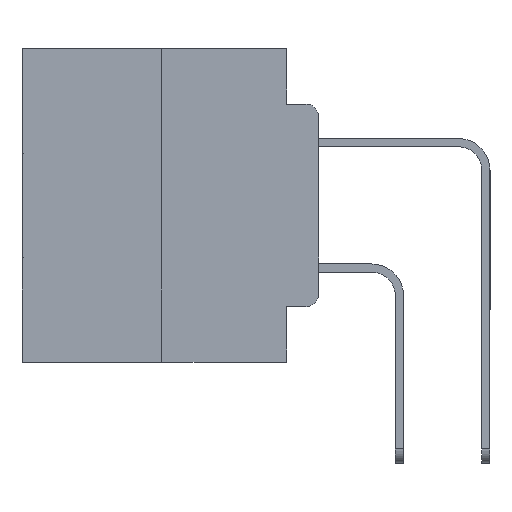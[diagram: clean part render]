
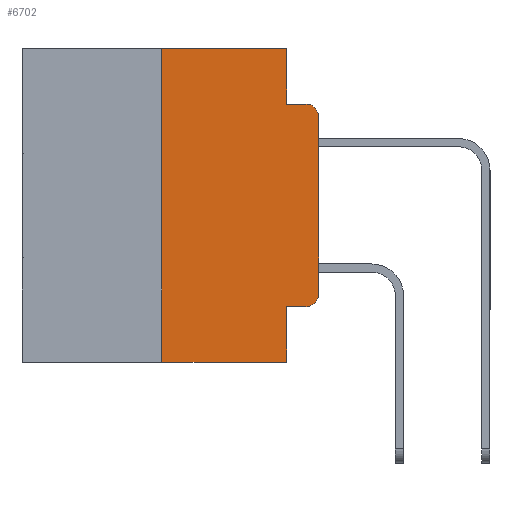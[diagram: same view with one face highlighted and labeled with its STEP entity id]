
A CAD part, left-side view. The second image highlights one B-rep face of the part: STEP entity #6702.
In plain terms, the highlighted planar face has unit normal (-1, 0, 0).
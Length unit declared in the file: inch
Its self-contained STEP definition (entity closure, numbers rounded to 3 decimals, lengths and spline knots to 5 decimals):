
#354 = LINE ( 'NONE', #2842, #5810 ) ;
#876 = VERTEX_POINT ( 'NONE', #20255 ) ;
#1134 = VERTEX_POINT ( 'NONE', #22027 ) ;
#1243 = DIRECTION ( 'NONE',  ( 0., 0., -1. ) ) ;
#1368 = ORIENTED_EDGE ( 'NONE', *, *, #16579, .T. ) ;
#1604 = VERTEX_POINT ( 'NONE', #1978 ) ;
#1875 = EDGE_CURVE ( 'NONE', #1134, #14332, #24399, .T. ) ;
#1978 = CARTESIAN_POINT ( 'NONE',  ( 0., 0., -0.1085 ) ) ;
#2536 = DIRECTION ( 'NONE',  ( 0., -1., 0. ) ) ;
#2578 = DIRECTION ( 'NONE',  ( -1., 0., 0. ) ) ;
#2840 = LINE ( 'NONE', #14932, #3560 ) ;
#2842 = CARTESIAN_POINT ( 'NONE',  ( 0., 0.25, 0. ) ) ;
#3298 = VERTEX_POINT ( 'NONE', #11558 ) ;
#3542 = LINE ( 'NONE', #20896, #20850 ) ;
#3560 = VECTOR ( 'NONE', #1243, 39.37008 ) ;
#4922 = DIRECTION ( 'NONE',  ( -1., 0., 0. ) ) ;
#5497 = CARTESIAN_POINT ( 'NONE',  ( 0., 0.25, -0.5 ) ) ;
#5541 = LINE ( 'NONE', #6587, #11650 ) ;
#5810 = VECTOR ( 'NONE', #20916, 39.37008 ) ;
#6446 = CARTESIAN_POINT ( 'NONE',  ( 0., 0.473, 0. ) ) ;
#6587 = CARTESIAN_POINT ( 'NONE',  ( 0., 0.473, -0.5 ) ) ;
#6595 = EDGE_LOOP ( 'NONE', ( #9119, #9317, #10600, #10644, #10692, #11097, #11295, #11640, #12481, #1368 ) ) ;
#6702 = ADVANCED_FACE ( 'NONE', ( #7708 ), #19922, .F. ) ;
#6956 = VERTEX_POINT ( 'NONE', #16199 ) ;
#7566 = CARTESIAN_POINT ( 'NONE',  ( 0., 0.051, 0. ) ) ;
#7708 = FACE_OUTER_BOUND ( 'NONE', #6595, .T. ) ;
#7837 = CIRCLE ( 'NONE', #10023, 0.02 ) ;
#8358 = DIRECTION ( 'NONE',  ( 0., -1., 0. ) ) ;
#8380 = CIRCLE ( 'NONE', #24462, 0.02 ) ;
#8742 = DIRECTION ( 'NONE',  ( 1., 0., 0. ) ) ;
#8753 = VECTOR ( 'NONE', #8358, 39.37008 ) ;
#8988 = CARTESIAN_POINT ( 'NONE',  ( 0., 0.02, -0.4115 ) ) ;
#9119 = ORIENTED_EDGE ( 'NONE', *, *, #19503, .T. ) ;
#9317 = ORIENTED_EDGE ( 'NONE', *, *, #23948, .T. ) ;
#9706 = EDGE_CURVE ( 'NONE', #6956, #23032, #26951, .T. ) ;
#10023 = AXIS2_PLACEMENT_3D ( 'NONE', #18459, #4922, #20680 ) ;
#10600 = ORIENTED_EDGE ( 'NONE', *, *, #1875, .F. ) ;
#10644 = ORIENTED_EDGE ( 'NONE', *, *, #23243, .F. ) ;
#10692 = ORIENTED_EDGE ( 'NONE', *, *, #16311, .F. ) ;
#11097 = ORIENTED_EDGE ( 'NONE', *, *, #17299, .F. ) ;
#11256 = CARTESIAN_POINT ( 'NONE',  ( 0., 0.02, -0.0885 ) ) ;
#11295 = ORIENTED_EDGE ( 'NONE', *, *, #15762, .T. ) ;
#11558 = CARTESIAN_POINT ( 'NONE',  ( 0., 0., -0.3915 ) ) ;
#11640 = ORIENTED_EDGE ( 'NONE', *, *, #22144, .F. ) ;
#11650 = VECTOR ( 'NONE', #28838, 39.37008 ) ;
#12117 = VERTEX_POINT ( 'NONE', #7566 ) ;
#12465 = VERTEX_POINT ( 'NONE', #17974 ) ;
#12481 = ORIENTED_EDGE ( 'NONE', *, *, #9706, .T. ) ;
#13220 = DIRECTION ( 'NONE',  ( 0., 0., 1. ) ) ;
#14332 = VERTEX_POINT ( 'NONE', #11256 ) ;
#14732 = LINE ( 'NONE', #23986, #8753 ) ;
#14932 = CARTESIAN_POINT ( 'NONE',  ( 0., 0.051, 0. ) ) ;
#15128 = VECTOR ( 'NONE', #13220, 39.37008 ) ;
#15160 = VECTOR ( 'NONE', #2536, 39.37008 ) ;
#15318 = DIRECTION ( 'NONE',  ( 0., -1., 0. ) ) ;
#15352 = CARTESIAN_POINT ( 'NONE',  ( 0., 0.051, -0.0885 ) ) ;
#15433 = CARTESIAN_POINT ( 'NONE',  ( 0., 0., 0. ) ) ;
#15762 = EDGE_CURVE ( 'NONE', #18158, #876, #5541, .T. ) ;
#15831 = LINE ( 'NONE', #15433, #15128 ) ;
#16199 = CARTESIAN_POINT ( 'NONE',  ( 0., 0.051, -0.4115 ) ) ;
#16208 = CARTESIAN_POINT ( 'NONE',  ( 0., 0.02, -0.3915 ) ) ;
#16311 = EDGE_CURVE ( 'NONE', #12465, #12117, #14732, .T. ) ;
#16579 = EDGE_CURVE ( 'NONE', #23032, #3298, #8380, .T. ) ;
#17299 = EDGE_CURVE ( 'NONE', #18158, #12465, #354, .T. ) ;
#17974 = CARTESIAN_POINT ( 'NONE',  ( 0., 0.25, 0. ) ) ;
#18158 = VERTEX_POINT ( 'NONE', #5497 ) ;
#18450 = DIRECTION ( 'NONE',  ( 0., 0., -1. ) ) ;
#18459 = CARTESIAN_POINT ( 'NONE',  ( 0., 0.02, -0.1085 ) ) ;
#19209 = VECTOR ( 'NONE', #15318, 39.37008 ) ;
#19503 = EDGE_CURVE ( 'NONE', #3298, #1604, #15831, .T. ) ;
#19922 = PLANE ( 'NONE',  #25377 ) ;
#20255 = CARTESIAN_POINT ( 'NONE',  ( 0., 0.051, -0.5 ) ) ;
#20680 = DIRECTION ( 'NONE',  ( 0., 0., -1. ) ) ;
#20850 = VECTOR ( 'NONE', #20996, 39.37008 ) ;
#20896 = CARTESIAN_POINT ( 'NONE',  ( 0., 0.051, 0. ) ) ;
#20916 = DIRECTION ( 'NONE',  ( 0., 0., 1. ) ) ;
#20996 = DIRECTION ( 'NONE',  ( 0., 0., -1. ) ) ;
#22027 = CARTESIAN_POINT ( 'NONE',  ( 0., 0.051, -0.0885 ) ) ;
#22144 = EDGE_CURVE ( 'NONE', #6956, #876, #2840, .T. ) ;
#23032 = VERTEX_POINT ( 'NONE', #8988 ) ;
#23243 = EDGE_CURVE ( 'NONE', #12117, #1134, #3542, .T. ) ;
#23948 = EDGE_CURVE ( 'NONE', #1604, #14332, #7837, .T. ) ;
#23986 = CARTESIAN_POINT ( 'NONE',  ( 0., 0.473, 0. ) ) ;
#24369 = DIRECTION ( 'NONE',  ( 0., 0., -1. ) ) ;
#24399 = LINE ( 'NONE', #15352, #19209 ) ;
#24462 = AXIS2_PLACEMENT_3D ( 'NONE', #16208, #2578, #18450 ) ;
#25377 = AXIS2_PLACEMENT_3D ( 'NONE', #6446, #8742, #24369 ) ;
#26951 = LINE ( 'NONE', #27216, #15160 ) ;
#27216 = CARTESIAN_POINT ( 'NONE',  ( 0., 0.051, -0.4115 ) ) ;
#28838 = DIRECTION ( 'NONE',  ( 0., -1., 0. ) ) ;
